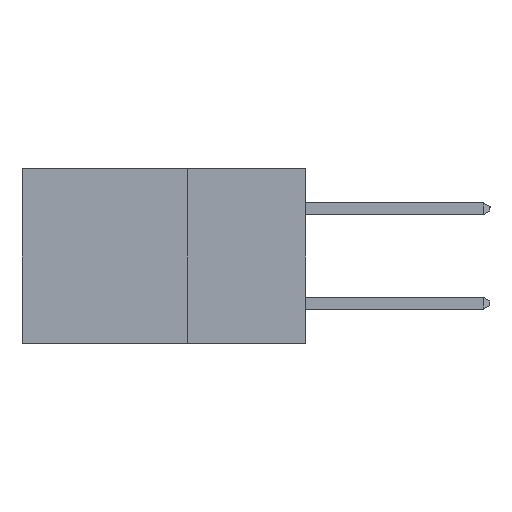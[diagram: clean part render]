
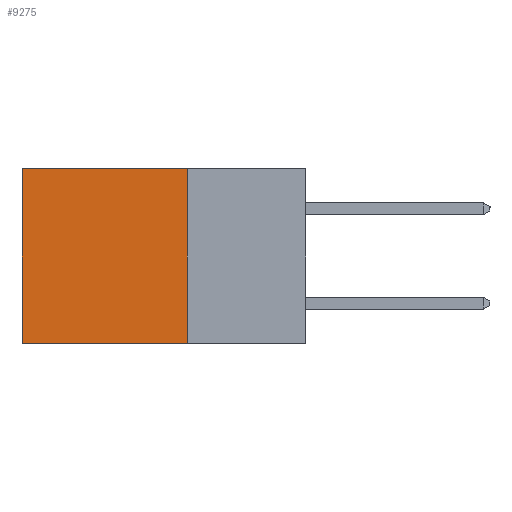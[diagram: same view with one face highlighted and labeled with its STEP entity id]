
A CAD part, left-side view. The second image highlights one B-rep face of the part: STEP entity #9275.
In plain terms, the highlighted planar face has unit normal (-1, 0, 0).
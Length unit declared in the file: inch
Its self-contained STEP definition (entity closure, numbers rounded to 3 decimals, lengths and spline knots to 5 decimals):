
#284 = ORIENTED_EDGE ( 'NONE', *, *, #7088, .F. ) ;
#748 = CARTESIAN_POINT ( 'NONE',  ( 0.2615, 0.6, 0. ) ) ;
#1026 = CARTESIAN_POINT ( 'NONE',  ( 0.2615, 0.25, -0.37 ) ) ;
#1227 = LINE ( 'NONE', #13524, #12824 ) ;
#1353 = LINE ( 'NONE', #3786, #5718 ) ;
#1579 = AXIS2_PLACEMENT_3D ( 'NONE', #1026, #5543, #7919 ) ;
#1700 = DIRECTION ( 'NONE',  ( 0., 0., -1. ) ) ;
#3101 = VECTOR ( 'NONE', #1700, 39.37008 ) ;
#3751 = VERTEX_POINT ( 'NONE', #10634 ) ;
#3786 = CARTESIAN_POINT ( 'NONE',  ( 0.2615, 0.25, -0.37 ) ) ;
#3914 = CARTESIAN_POINT ( 'NONE',  ( 0.2615, 0.6, -0.37 ) ) ;
#4713 = ORIENTED_EDGE ( 'NONE', *, *, #13715, .T. ) ;
#5167 = ORIENTED_EDGE ( 'NONE', *, *, #9865, .F. ) ;
#5543 = DIRECTION ( 'NONE',  ( 1., 0., 0. ) ) ;
#5718 = VECTOR ( 'NONE', #12896, 39.37008 ) ;
#6093 = CARTESIAN_POINT ( 'NONE',  ( 0.2615, 0.25, -0.37 ) ) ;
#6752 = CARTESIAN_POINT ( 'NONE',  ( 0.2615, 0.25, 0. ) ) ;
#7088 = EDGE_CURVE ( 'NONE', #7231, #3751, #12958, .T. ) ;
#7187 = VERTEX_POINT ( 'NONE', #748 ) ;
#7231 = VERTEX_POINT ( 'NONE', #6752 ) ;
#7364 = EDGE_CURVE ( 'NONE', #7187, #13841, #11970, .T. ) ;
#7919 = DIRECTION ( 'NONE',  ( 0., 0., -1. ) ) ;
#8087 = VECTOR ( 'NONE', #12817, 39.37008 ) ;
#9275 = ADVANCED_FACE ( 'NONE', ( #13454 ), #13612, .F. ) ;
#9865 = EDGE_CURVE ( 'NONE', #3751, #13841, #1353, .T. ) ;
#10634 = CARTESIAN_POINT ( 'NONE',  ( 0.2615, 0.25, -0.37 ) ) ;
#10836 = ORIENTED_EDGE ( 'NONE', *, *, #7364, .T. ) ;
#11970 = LINE ( 'NONE', #3914, #3101 ) ;
#12260 = DIRECTION ( 'NONE',  ( 0., 1., 0. ) ) ;
#12329 = CARTESIAN_POINT ( 'NONE',  ( 0.2615, 0.6, -0.37 ) ) ;
#12584 = EDGE_LOOP ( 'NONE', ( #10836, #5167, #284, #4713 ) ) ;
#12817 = DIRECTION ( 'NONE',  ( 0., 0., -1. ) ) ;
#12824 = VECTOR ( 'NONE', #12260, 39.37008 ) ;
#12896 = DIRECTION ( 'NONE',  ( 0., 1., 0. ) ) ;
#12958 = LINE ( 'NONE', #6093, #8087 ) ;
#13454 = FACE_OUTER_BOUND ( 'NONE', #12584, .T. ) ;
#13524 = CARTESIAN_POINT ( 'NONE',  ( 0.2615, 0.25, 0. ) ) ;
#13612 = PLANE ( 'NONE',  #1579 ) ;
#13715 = EDGE_CURVE ( 'NONE', #7231, #7187, #1227, .T. ) ;
#13841 = VERTEX_POINT ( 'NONE', #12329 ) ;
